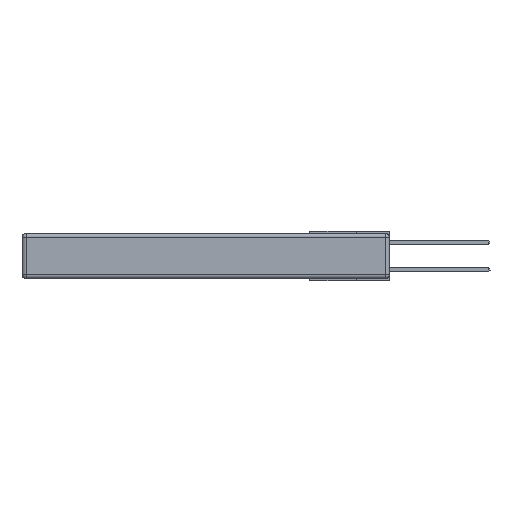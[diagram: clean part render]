
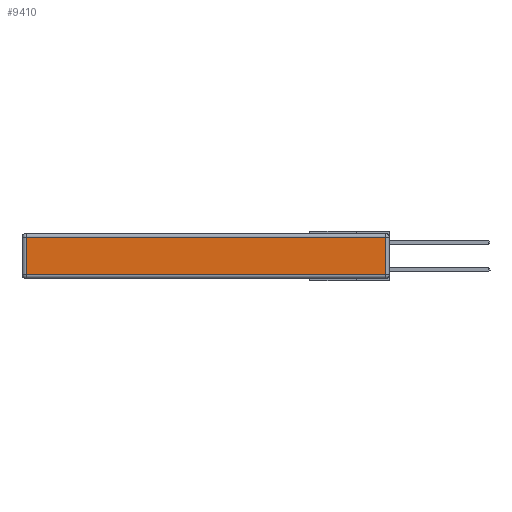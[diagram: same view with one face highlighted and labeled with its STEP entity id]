
A CAD part, left-side view. The second image highlights one B-rep face of the part: STEP entity #9410.
In plain terms, the highlighted planar face has unit normal (-1, 0, 0).
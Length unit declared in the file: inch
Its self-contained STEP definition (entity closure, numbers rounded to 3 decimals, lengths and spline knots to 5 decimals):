
#682 = FACE_OUTER_BOUND ( 'NONE', #3696, .T. ) ;
#1144 = VERTEX_POINT ( 'NONE', #6037 ) ;
#1360 = VERTEX_POINT ( 'NONE', #4730 ) ;
#1579 = LINE ( 'NONE', #11432, #8255 ) ;
#1667 = DIRECTION ( 'NONE',  ( 0., 1., 0. ) ) ;
#3696 = EDGE_LOOP ( 'NONE', ( #16490, #15862, #9307, #9573 ) ) ;
#3844 = DIRECTION ( 'NONE',  ( -1., 0., 0. ) ) ;
#4005 = LINE ( 'NONE', #9039, #10898 ) ;
#4365 = VECTOR ( 'NONE', #5297, 39.37008 ) ;
#4730 = CARTESIAN_POINT ( 'NONE',  ( 0., 0.03, -0.313 ) ) ;
#5292 = EDGE_CURVE ( 'NONE', #1144, #16801, #17368, .T. ) ;
#5297 = DIRECTION ( 'NONE',  ( 0., 0., -1. ) ) ;
#5338 = DIRECTION ( 'NONE',  ( 0., 0., 1. ) ) ;
#5816 = CARTESIAN_POINT ( 'NONE',  ( 0., 2.75, -0.03 ) ) ;
#6037 = CARTESIAN_POINT ( 'NONE',  ( 0., 0.03, -0.03 ) ) ;
#7750 = VECTOR ( 'NONE', #1667, 39.37008 ) ;
#8175 = CARTESIAN_POINT ( 'NONE',  ( 0., 0., -0.343 ) ) ;
#8255 = VECTOR ( 'NONE', #12869, 39.37008 ) ;
#8395 = CARTESIAN_POINT ( 'NONE',  ( 0., 2.72, -0.03 ) ) ;
#9039 = CARTESIAN_POINT ( 'NONE',  ( 0., 0., -0.313 ) ) ;
#9101 = DIRECTION ( 'NONE',  ( 0., -1., 0. ) ) ;
#9307 = ORIENTED_EDGE ( 'NONE', *, *, #5292, .T. ) ;
#9410 = ADVANCED_FACE ( 'NONE', ( #682 ), #10785, .T. ) ;
#9573 = ORIENTED_EDGE ( 'NONE', *, *, #9887, .T. ) ;
#9887 = EDGE_CURVE ( 'NONE', #16801, #13581, #18568, .T. ) ;
#10033 = EDGE_CURVE ( 'NONE', #1360, #1144, #1579, .T. ) ;
#10785 = PLANE ( 'NONE',  #16943 ) ;
#10898 = VECTOR ( 'NONE', #9101, 39.37008 ) ;
#11274 = CARTESIAN_POINT ( 'NONE',  ( 0., 2.72, -0.313 ) ) ;
#11432 = CARTESIAN_POINT ( 'NONE',  ( 0., 0.03, -0.343 ) ) ;
#12353 = EDGE_CURVE ( 'NONE', #13581, #1360, #4005, .T. ) ;
#12869 = DIRECTION ( 'NONE',  ( 0., 0., 1. ) ) ;
#13581 = VERTEX_POINT ( 'NONE', #11274 ) ;
#15862 = ORIENTED_EDGE ( 'NONE', *, *, #10033, .T. ) ;
#16490 = ORIENTED_EDGE ( 'NONE', *, *, #12353, .T. ) ;
#16801 = VERTEX_POINT ( 'NONE', #8395 ) ;
#16943 = AXIS2_PLACEMENT_3D ( 'NONE', #8175, #3844, #5338 ) ;
#17104 = CARTESIAN_POINT ( 'NONE',  ( 0., 2.72, -0.343 ) ) ;
#17368 = LINE ( 'NONE', #5816, #7750 ) ;
#18568 = LINE ( 'NONE', #17104, #4365 ) ;
